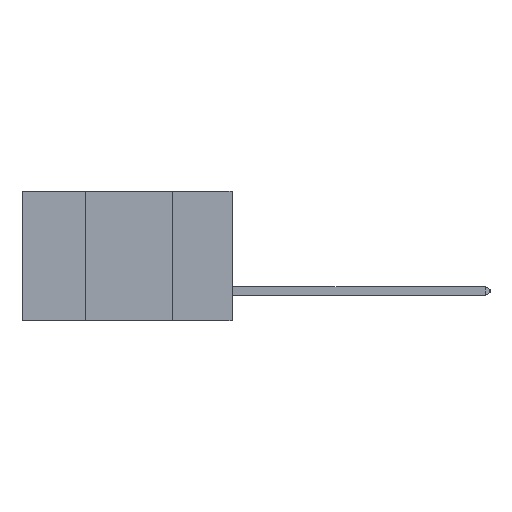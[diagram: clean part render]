
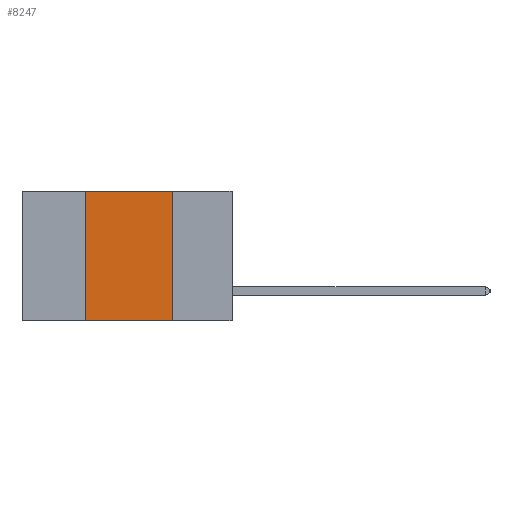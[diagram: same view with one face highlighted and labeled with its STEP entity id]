
A CAD part, left-side view. The second image highlights one B-rep face of the part: STEP entity #8247.
In plain terms, the highlighted planar face has unit normal (-1, 0, 0).
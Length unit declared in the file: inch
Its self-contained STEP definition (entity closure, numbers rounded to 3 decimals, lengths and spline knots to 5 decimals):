
#161 = EDGE_CURVE ( 'NONE', #10326, #9755, #14326, .T. ) ;
#1116 = DIRECTION ( 'NONE',  ( 0., -1., 0. ) ) ;
#1881 = DIRECTION ( 'NONE',  ( 0., 0., 1. ) ) ;
#2867 = LINE ( 'NONE', #6453, #18616 ) ;
#3307 = DIRECTION ( 'NONE',  ( 0., 0., -1. ) ) ;
#3671 = CARTESIAN_POINT ( 'NONE',  ( 0., 0.17, -0.37 ) ) ;
#3738 = EDGE_LOOP ( 'NONE', ( #15077, #8887, #15757, #8970 ) ) ;
#4518 = AXIS2_PLACEMENT_3D ( 'NONE', #13279, #8905, #19045 ) ;
#4868 = CARTESIAN_POINT ( 'NONE',  ( 0., 0.42, 0. ) ) ;
#6379 = CARTESIAN_POINT ( 'NONE',  ( 0., 0.6, -0.37 ) ) ;
#6453 = CARTESIAN_POINT ( 'NONE',  ( 0., 0.17, 0. ) ) ;
#6518 = CARTESIAN_POINT ( 'NONE',  ( 0., 0.17, 0. ) ) ;
#6531 = VECTOR ( 'NONE', #17615, 39.37008 ) ;
#6594 = CARTESIAN_POINT ( 'NONE',  ( 0., 0.42, -0.37 ) ) ;
#7537 = EDGE_CURVE ( 'NONE', #13119, #18326, #7781, .T. ) ;
#7781 = LINE ( 'NONE', #10258, #15131 ) ;
#8247 = ADVANCED_FACE ( 'NONE', ( #11722 ), #17646, .F. ) ;
#8887 = ORIENTED_EDGE ( 'NONE', *, *, #7537, .F. ) ;
#8905 = DIRECTION ( 'NONE',  ( 1., 0., 0. ) ) ;
#8970 = ORIENTED_EDGE ( 'NONE', *, *, #161, .T. ) ;
#8984 = EDGE_CURVE ( 'NONE', #10326, #13119, #17359, .T. ) ;
#9755 = VERTEX_POINT ( 'NONE', #3671 ) ;
#10258 = CARTESIAN_POINT ( 'NONE',  ( 0., 0.6, 0. ) ) ;
#10326 = VERTEX_POINT ( 'NONE', #6594 ) ;
#10697 = EDGE_CURVE ( 'NONE', #18326, #9755, #2867, .T. ) ;
#11722 = FACE_OUTER_BOUND ( 'NONE', #3738, .T. ) ;
#13119 = VERTEX_POINT ( 'NONE', #4868 ) ;
#13279 = CARTESIAN_POINT ( 'NONE',  ( 0., 0.6, 0. ) ) ;
#14326 = LINE ( 'NONE', #6379, #6531 ) ;
#15077 = ORIENTED_EDGE ( 'NONE', *, *, #10697, .F. ) ;
#15131 = VECTOR ( 'NONE', #1116, 39.37008 ) ;
#15300 = CARTESIAN_POINT ( 'NONE',  ( 0., 0.42, 0. ) ) ;
#15757 = ORIENTED_EDGE ( 'NONE', *, *, #8984, .F. ) ;
#17359 = LINE ( 'NONE', #15300, #18253 ) ;
#17615 = DIRECTION ( 'NONE',  ( 0., -1., 0. ) ) ;
#17646 = PLANE ( 'NONE',  #4518 ) ;
#18253 = VECTOR ( 'NONE', #1881, 39.37008 ) ;
#18326 = VERTEX_POINT ( 'NONE', #6518 ) ;
#18616 = VECTOR ( 'NONE', #3307, 39.37008 ) ;
#19045 = DIRECTION ( 'NONE',  ( 0., 0., -1. ) ) ;
